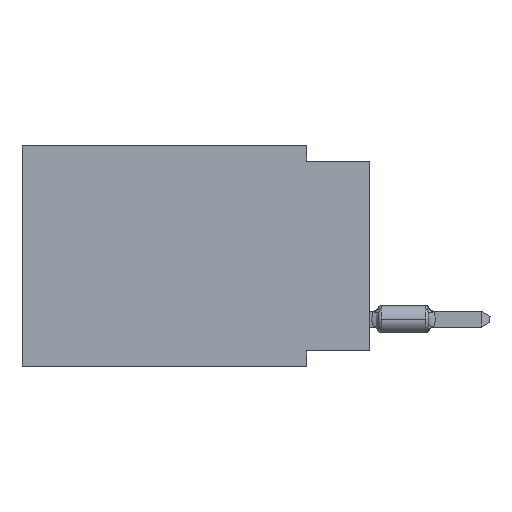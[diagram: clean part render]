
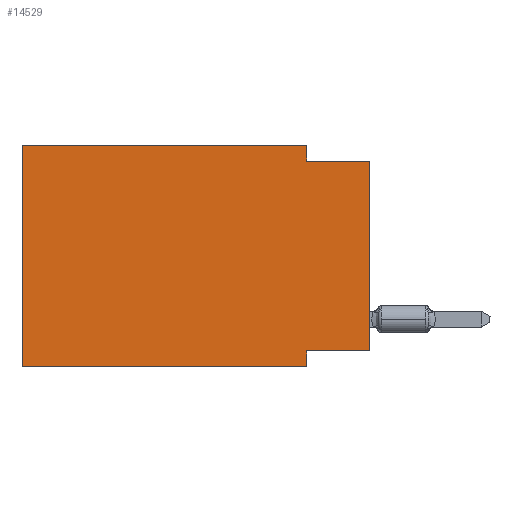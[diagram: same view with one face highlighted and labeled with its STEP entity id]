
A CAD part, left-side view. The second image highlights one B-rep face of the part: STEP entity #14529.
In plain terms, the highlighted planar face has unit normal (-1, 0, 0).
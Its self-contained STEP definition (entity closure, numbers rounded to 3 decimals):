
#1579 = DIRECTION ( 'NONE',  ( 0., 0., 1. ) ) ;
#1823 = VECTOR ( 'NONE', #19716, 1000. ) ;
#2908 = ORIENTED_EDGE ( 'NONE', *, *, #21009, .F. ) ;
#3157 = EDGE_CURVE ( 'NONE', #49200, #10377, #33556, .T. ) ;
#4181 = LINE ( 'NONE', #8201, #1823 ) ;
#4716 = ORIENTED_EDGE ( 'NONE', *, *, #30615, .F. ) ;
#4859 = VECTOR ( 'NONE', #14213, 1000. ) ;
#6574 = EDGE_CURVE ( 'NONE', #11346, #39233, #22811, .T. ) ;
#7225 = CARTESIAN_POINT ( 'NONE',  ( 0., 0., 0. ) ) ;
#7362 = VECTOR ( 'NONE', #7952, 1000. ) ;
#7952 = DIRECTION ( 'NONE',  ( 0., -1., 0. ) ) ;
#8201 = CARTESIAN_POINT ( 'NONE',  ( 0., 2.54, 0. ) ) ;
#9102 = CARTESIAN_POINT ( 'NONE',  ( 0., 13.97, 0. ) ) ;
#10201 = AXIS2_PLACEMENT_3D ( 'NONE', #12591, #16596, #40204 ) ;
#10377 = VERTEX_POINT ( 'NONE', #22573 ) ;
#10491 = VECTOR ( 'NONE', #11059, 1000. ) ;
#11059 = DIRECTION ( 'NONE',  ( 0., 1., 0. ) ) ;
#11346 = VERTEX_POINT ( 'NONE', #15617 ) ;
#12591 = CARTESIAN_POINT ( 'NONE',  ( 0., 13.97, 0. ) ) ;
#13110 = LINE ( 'NONE', #9102, #44071 ) ;
#13327 = FACE_OUTER_BOUND ( 'NONE', #34528, .T. ) ;
#14213 = DIRECTION ( 'NONE',  ( 0., -1., 0. ) ) ;
#14280 = CARTESIAN_POINT ( 'NONE',  ( 0., 2.54, -8.89 ) ) ;
#14529 = ADVANCED_FACE ( 'NONE', ( #13327 ), #27913, .F. ) ;
#15286 = DIRECTION ( 'NONE',  ( 0., -1., 0. ) ) ;
#15335 = ORIENTED_EDGE ( 'NONE', *, *, #22117, .F. ) ;
#15617 = CARTESIAN_POINT ( 'NONE',  ( 0., 2.54, -0.635 ) ) ;
#16596 = DIRECTION ( 'NONE',  ( 1., 0., 0. ) ) ;
#16893 = CARTESIAN_POINT ( 'NONE',  ( 0., 2.54, -8.255 ) ) ;
#19716 = DIRECTION ( 'NONE',  ( 0., 0., -1. ) ) ;
#19813 = ORIENTED_EDGE ( 'NONE', *, *, #3157, .F. ) ;
#20604 = EDGE_CURVE ( 'NONE', #41344, #29949, #34056, .T. ) ;
#21009 = EDGE_CURVE ( 'NONE', #10377, #11346, #4181, .T. ) ;
#22117 = EDGE_CURVE ( 'NONE', #41566, #29949, #25591, .T. ) ;
#22304 = CARTESIAN_POINT ( 'NONE',  ( 0., 0., -0.635 ) ) ;
#22573 = CARTESIAN_POINT ( 'NONE',  ( 0., 2.54, 0. ) ) ;
#22642 = ORIENTED_EDGE ( 'NONE', *, *, #37533, .T. ) ;
#22811 = LINE ( 'NONE', #22304, #35727 ) ;
#23967 = CARTESIAN_POINT ( 'NONE',  ( 0., 0., -0.635 ) ) ;
#25591 = LINE ( 'NONE', #14280, #28329 ) ;
#25779 = VECTOR ( 'NONE', #30577, 1000. ) ;
#27913 = PLANE ( 'NONE',  #10201 ) ;
#28329 = VECTOR ( 'NONE', #44930, 1000. ) ;
#29949 = VERTEX_POINT ( 'NONE', #30322 ) ;
#30158 = CARTESIAN_POINT ( 'NONE',  ( 0., 0., -8.255 ) ) ;
#30322 = CARTESIAN_POINT ( 'NONE',  ( 0., 2.54, -8.89 ) ) ;
#30408 = LINE ( 'NONE', #30158, #10491 ) ;
#30577 = DIRECTION ( 'NONE',  ( 0., 0., 1. ) ) ;
#30615 = EDGE_CURVE ( 'NONE', #41344, #49200, #13110, .T. ) ;
#31041 = CARTESIAN_POINT ( 'NONE',  ( 0., 13.97, -8.89 ) ) ;
#31187 = CARTESIAN_POINT ( 'NONE',  ( 0., 0., -8.255 ) ) ;
#31733 = ORIENTED_EDGE ( 'NONE', *, *, #20604, .T. ) ;
#32784 = EDGE_CURVE ( 'NONE', #44948, #41566, #30408, .T. ) ;
#33556 = LINE ( 'NONE', #44379, #4859 ) ;
#33844 = LINE ( 'NONE', #7225, #25779 ) ;
#33858 = ORIENTED_EDGE ( 'NONE', *, *, #6574, .F. ) ;
#34056 = LINE ( 'NONE', #31041, #7362 ) ;
#34528 = EDGE_LOOP ( 'NONE', ( #22642, #33858, #2908, #19813, #4716, #31733, #15335, #40766 ) ) ;
#35727 = VECTOR ( 'NONE', #15286, 1000. ) ;
#37533 = EDGE_CURVE ( 'NONE', #44948, #39233, #33844, .T. ) ;
#39233 = VERTEX_POINT ( 'NONE', #23967 ) ;
#40204 = DIRECTION ( 'NONE',  ( 0., 0., -1. ) ) ;
#40766 = ORIENTED_EDGE ( 'NONE', *, *, #32784, .F. ) ;
#40789 = CARTESIAN_POINT ( 'NONE',  ( 0., 13.97, -8.89 ) ) ;
#41344 = VERTEX_POINT ( 'NONE', #40789 ) ;
#41566 = VERTEX_POINT ( 'NONE', #16893 ) ;
#44071 = VECTOR ( 'NONE', #1579, 1000. ) ;
#44379 = CARTESIAN_POINT ( 'NONE',  ( 0., 13.97, 0. ) ) ;
#44930 = DIRECTION ( 'NONE',  ( 0., 0., -1. ) ) ;
#44948 = VERTEX_POINT ( 'NONE', #31187 ) ;
#46734 = CARTESIAN_POINT ( 'NONE',  ( 0., 13.97, 0. ) ) ;
#49200 = VERTEX_POINT ( 'NONE', #46734 ) ;
